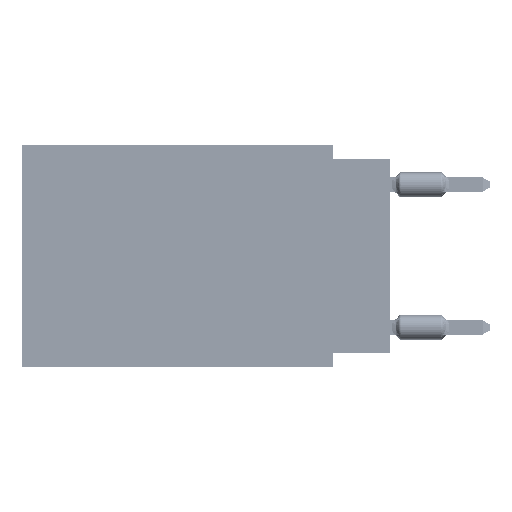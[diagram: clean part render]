
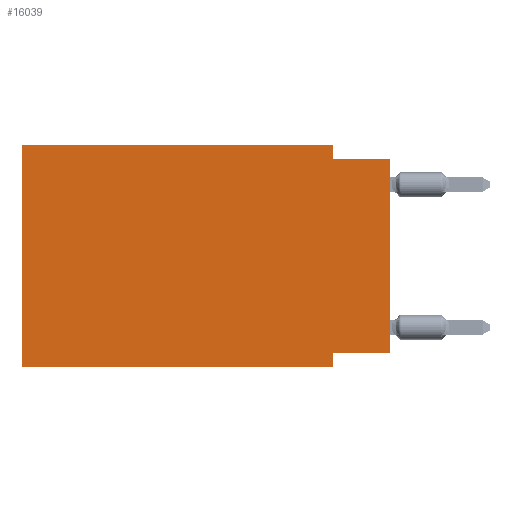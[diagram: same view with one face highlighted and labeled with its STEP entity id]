
A CAD part, left-side view. The second image highlights one B-rep face of the part: STEP entity #16039.
In plain terms, the highlighted planar face has unit normal (-1, 0, 0).
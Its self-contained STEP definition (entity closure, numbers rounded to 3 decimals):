
#286 = CARTESIAN_POINT ( 'NONE',  ( 0., 16.383, 0. ) ) ;
#337 = AXIS2_PLACEMENT_3D ( 'NONE', #24249, #69080, #2761 ) ;
#1168 = VERTEX_POINT ( 'NONE', #18382 ) ;
#2287 = EDGE_LOOP ( 'NONE', ( #52356, #34931, #51624, #38104, #48749, #55054, #22443, #4297 ) ) ;
#2434 = CARTESIAN_POINT ( 'NONE',  ( 0., 2.54, -9.906 ) ) ;
#2589 = CARTESIAN_POINT ( 'NONE',  ( 0., 2.54, 0. ) ) ;
#2761 = DIRECTION ( 'NONE',  ( 0., 0., -1. ) ) ;
#2943 = VECTOR ( 'NONE', #52217, 1000. ) ;
#4297 = ORIENTED_EDGE ( 'NONE', *, *, #20617, .F. ) ;
#4392 = EDGE_CURVE ( 'NONE', #17246, #1168, #57500, .T. ) ;
#4492 = DIRECTION ( 'NONE',  ( 0., 0., -1. ) ) ;
#4890 = CARTESIAN_POINT ( 'NONE',  ( 0., 0., 0. ) ) ;
#8146 = CARTESIAN_POINT ( 'NONE',  ( 0., 2.54, -9.271 ) ) ;
#8409 = CARTESIAN_POINT ( 'NONE',  ( 0., 0., -9.271 ) ) ;
#8420 = DIRECTION ( 'NONE',  ( 0., 0., -1. ) ) ;
#9052 = EDGE_CURVE ( 'NONE', #59255, #1168, #54411, .T. ) ;
#9356 = VECTOR ( 'NONE', #69280, 1000. ) ;
#9490 = CARTESIAN_POINT ( 'NONE',  ( 0., 16.383, 0. ) ) ;
#10987 = VECTOR ( 'NONE', #58961, 1000. ) ;
#11466 = EDGE_CURVE ( 'NONE', #16889, #19619, #48981, .T. ) ;
#12043 = CARTESIAN_POINT ( 'NONE',  ( 0., 0., -0.635 ) ) ;
#14241 = LINE ( 'NONE', #2589, #54547 ) ;
#16039 = ADVANCED_FACE ( 'NONE', ( #53054 ), #51593, .F. ) ;
#16753 = VERTEX_POINT ( 'NONE', #46648 ) ;
#16889 = VERTEX_POINT ( 'NONE', #8409 ) ;
#17246 = VERTEX_POINT ( 'NONE', #68060 ) ;
#18382 = CARTESIAN_POINT ( 'NONE',  ( 0., 2.54, -9.906 ) ) ;
#19619 = VERTEX_POINT ( 'NONE', #22628 ) ;
#20320 = VECTOR ( 'NONE', #61245, 1000. ) ;
#20617 = EDGE_CURVE ( 'NONE', #16889, #59255, #57311, .T. ) ;
#22443 = ORIENTED_EDGE ( 'NONE', *, *, #9052, .F. ) ;
#22628 = CARTESIAN_POINT ( 'NONE',  ( 0., 0., -0.635 ) ) ;
#24249 = CARTESIAN_POINT ( 'NONE',  ( 0., 16.383, 0. ) ) ;
#31865 = DIRECTION ( 'NONE',  ( 0., 0., 1. ) ) ;
#33599 = VERTEX_POINT ( 'NONE', #57288 ) ;
#33787 = LINE ( 'NONE', #286, #68167 ) ;
#34931 = ORIENTED_EDGE ( 'NONE', *, *, #62615, .F. ) ;
#38104 = ORIENTED_EDGE ( 'NONE', *, *, #70386, .F. ) ;
#39278 = VERTEX_POINT ( 'NONE', #41023 ) ;
#41023 = CARTESIAN_POINT ( 'NONE',  ( 0., 16.383, 0. ) ) ;
#45438 = DIRECTION ( 'NONE',  ( 0., 0., 1. ) ) ;
#46648 = CARTESIAN_POINT ( 'NONE',  ( 0., 2.54, 0. ) ) ;
#47102 = CARTESIAN_POINT ( 'NONE',  ( 0., 0., -9.271 ) ) ;
#47287 = CARTESIAN_POINT ( 'NONE',  ( 0., 16.383, -9.906 ) ) ;
#48122 = EDGE_CURVE ( 'NONE', #17246, #39278, #33787, .T. ) ;
#48749 = ORIENTED_EDGE ( 'NONE', *, *, #48122, .F. ) ;
#48981 = LINE ( 'NONE', #4890, #68682 ) ;
#51593 = PLANE ( 'NONE',  #337 ) ;
#51624 = ORIENTED_EDGE ( 'NONE', *, *, #66570, .F. ) ;
#52217 = DIRECTION ( 'NONE',  ( 0., 1., 0. ) ) ;
#52356 = ORIENTED_EDGE ( 'NONE', *, *, #11466, .T. ) ;
#53054 = FACE_OUTER_BOUND ( 'NONE', #2287, .T. ) ;
#53506 = VECTOR ( 'NONE', #4492, 1000. ) ;
#54411 = LINE ( 'NONE', #2434, #53506 ) ;
#54547 = VECTOR ( 'NONE', #8420, 1000. ) ;
#55054 = ORIENTED_EDGE ( 'NONE', *, *, #4392, .T. ) ;
#57288 = CARTESIAN_POINT ( 'NONE',  ( 0., 2.54, -0.635 ) ) ;
#57311 = LINE ( 'NONE', #47102, #2943 ) ;
#57500 = LINE ( 'NONE', #47287, #10987 ) ;
#58305 = LINE ( 'NONE', #9490, #9356 ) ;
#58961 = DIRECTION ( 'NONE',  ( 0., -1., 0. ) ) ;
#59255 = VERTEX_POINT ( 'NONE', #8146 ) ;
#61245 = DIRECTION ( 'NONE',  ( 0., -1., 0. ) ) ;
#61942 = LINE ( 'NONE', #12043, #20320 ) ;
#62615 = EDGE_CURVE ( 'NONE', #33599, #19619, #61942, .T. ) ;
#66570 = EDGE_CURVE ( 'NONE', #16753, #33599, #14241, .T. ) ;
#68060 = CARTESIAN_POINT ( 'NONE',  ( 0., 16.383, -9.906 ) ) ;
#68167 = VECTOR ( 'NONE', #45438, 1000. ) ;
#68682 = VECTOR ( 'NONE', #31865, 1000. ) ;
#69080 = DIRECTION ( 'NONE',  ( 1., 0., 0. ) ) ;
#69280 = DIRECTION ( 'NONE',  ( 0., -1., 0. ) ) ;
#70386 = EDGE_CURVE ( 'NONE', #39278, #16753, #58305, .T. ) ;
